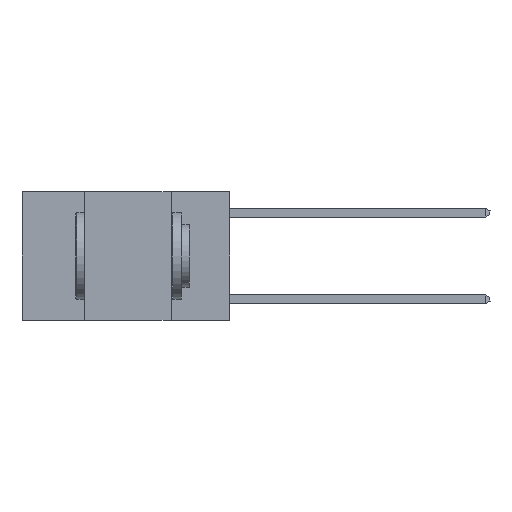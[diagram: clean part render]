
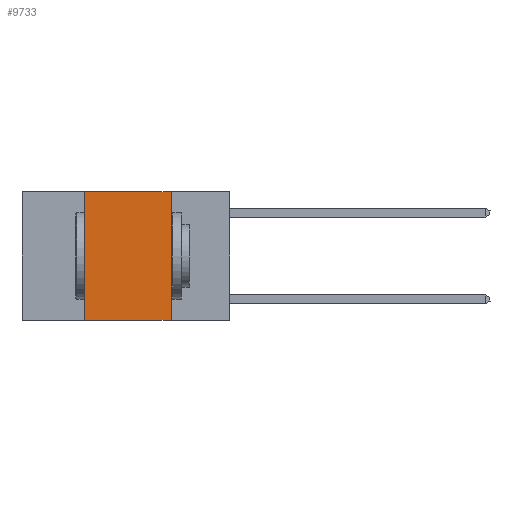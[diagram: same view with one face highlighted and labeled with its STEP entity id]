
A CAD part, left-side view. The second image highlights one B-rep face of the part: STEP entity #9733.
In plain terms, the highlighted planar face has unit normal (-1, 0, 0).
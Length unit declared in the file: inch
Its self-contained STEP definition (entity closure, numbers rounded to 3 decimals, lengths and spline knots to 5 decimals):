
#222 = CARTESIAN_POINT ( 'NONE',  ( 0., 0.17, -0.37 ) ) ;
#662 = CARTESIAN_POINT ( 'NONE',  ( 0., 0.6, -0.37 ) ) ;
#1721 = CARTESIAN_POINT ( 'NONE',  ( 0., 0.42, -0.37 ) ) ;
#1966 = ORIENTED_EDGE ( 'NONE', *, *, #8990, .F. ) ;
#2227 = VECTOR ( 'NONE', #8980, 39.37008 ) ;
#3041 = EDGE_CURVE ( 'NONE', #3963, #9474, #10736, .T. ) ;
#3168 = LINE ( 'NONE', #12725, #5947 ) ;
#3656 = EDGE_CURVE ( 'NONE', #4979, #4666, #3680, .T. ) ;
#3680 = LINE ( 'NONE', #12036, #11191 ) ;
#3963 = VERTEX_POINT ( 'NONE', #11449 ) ;
#4666 = VERTEX_POINT ( 'NONE', #6371 ) ;
#4731 = ORIENTED_EDGE ( 'NONE', *, *, #3656, .F. ) ;
#4768 = CARTESIAN_POINT ( 'NONE',  ( 0., 0.6, 0. ) ) ;
#4979 = VERTEX_POINT ( 'NONE', #1721 ) ;
#5627 = DIRECTION ( 'NONE',  ( 0., -1., 0. ) ) ;
#5796 = EDGE_CURVE ( 'NONE', #4979, #9474, #12087, .T. ) ;
#5799 = DIRECTION ( 'NONE',  ( 0., 0., -1. ) ) ;
#5947 = VECTOR ( 'NONE', #5627, 39.37008 ) ;
#6371 = CARTESIAN_POINT ( 'NONE',  ( 0., 0.42, 0. ) ) ;
#7450 = ORIENTED_EDGE ( 'NONE', *, *, #5796, .T. ) ;
#7848 = DIRECTION ( 'NONE',  ( 0., -1., 0. ) ) ;
#8469 = FACE_OUTER_BOUND ( 'NONE', #9484, .T. ) ;
#8493 = AXIS2_PLACEMENT_3D ( 'NONE', #4768, #11900, #5799 ) ;
#8980 = DIRECTION ( 'NONE',  ( 0., 0., -1. ) ) ;
#8990 = EDGE_CURVE ( 'NONE', #4666, #3963, #3168, .T. ) ;
#9474 = VERTEX_POINT ( 'NONE', #222 ) ;
#9484 = EDGE_LOOP ( 'NONE', ( #12518, #1966, #4731, #7450 ) ) ;
#9698 = VECTOR ( 'NONE', #7848, 39.37008 ) ;
#9733 = ADVANCED_FACE ( 'NONE', ( #8469 ), #10877, .F. ) ;
#10736 = LINE ( 'NONE', #10985, #2227 ) ;
#10877 = PLANE ( 'NONE',  #8493 ) ;
#10985 = CARTESIAN_POINT ( 'NONE',  ( 0., 0.17, 0. ) ) ;
#11191 = VECTOR ( 'NONE', #13011, 39.37008 ) ;
#11449 = CARTESIAN_POINT ( 'NONE',  ( 0., 0.17, 0. ) ) ;
#11900 = DIRECTION ( 'NONE',  ( 1., 0., 0. ) ) ;
#12036 = CARTESIAN_POINT ( 'NONE',  ( 0., 0.42, 0. ) ) ;
#12087 = LINE ( 'NONE', #662, #9698 ) ;
#12518 = ORIENTED_EDGE ( 'NONE', *, *, #3041, .F. ) ;
#12725 = CARTESIAN_POINT ( 'NONE',  ( 0., 0.6, 0. ) ) ;
#13011 = DIRECTION ( 'NONE',  ( 0., 0., 1. ) ) ;
